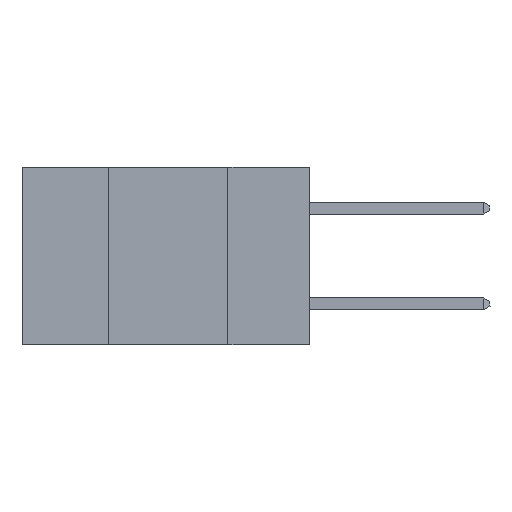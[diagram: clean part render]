
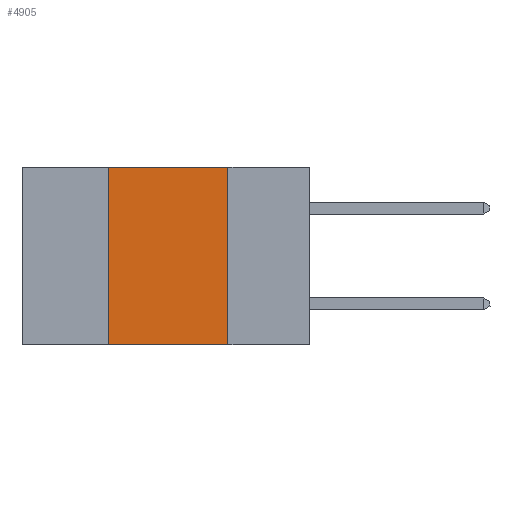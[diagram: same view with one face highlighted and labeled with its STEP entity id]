
A CAD part, left-side view. The second image highlights one B-rep face of the part: STEP entity #4905.
In plain terms, the highlighted planar face has unit normal (-1, 0, 0).
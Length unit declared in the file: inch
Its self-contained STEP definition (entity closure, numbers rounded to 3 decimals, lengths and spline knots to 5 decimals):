
#242 = FACE_OUTER_BOUND ( 'NONE', #3229, .T. ) ;
#1095 = CARTESIAN_POINT ( 'NONE',  ( 0., 0.42, 0. ) ) ;
#1418 = VERTEX_POINT ( 'NONE', #6916 ) ;
#1451 = CARTESIAN_POINT ( 'NONE',  ( 0., 0.42, 0. ) ) ;
#1574 = DIRECTION ( 'NONE',  ( 1., 0., 0. ) ) ;
#1758 = DIRECTION ( 'NONE',  ( 0., -1., 0. ) ) ;
#2388 = VERTEX_POINT ( 'NONE', #1095 ) ;
#2653 = DIRECTION ( 'NONE',  ( 0., -1., 0. ) ) ;
#3075 = LINE ( 'NONE', #4954, #3851 ) ;
#3144 = DIRECTION ( 'NONE',  ( 0., 0., -1. ) ) ;
#3229 = EDGE_LOOP ( 'NONE', ( #6020, #6443, #9209, #9977 ) ) ;
#3851 = VECTOR ( 'NONE', #2653, 39.37008 ) ;
#4242 = VERTEX_POINT ( 'NONE', #8302 ) ;
#4789 = EDGE_CURVE ( 'NONE', #5990, #1418, #3075, .T. ) ;
#4842 = EDGE_CURVE ( 'NONE', #4242, #1418, #7508, .T. ) ;
#4905 = ADVANCED_FACE ( 'NONE', ( #242 ), #10369, .F. ) ;
#4954 = CARTESIAN_POINT ( 'NONE',  ( 0., 0.6, -0.37 ) ) ;
#5072 = VECTOR ( 'NONE', #1758, 39.37008 ) ;
#5334 = DIRECTION ( 'NONE',  ( 0., 0., 1. ) ) ;
#5521 = CARTESIAN_POINT ( 'NONE',  ( 0., 0.6, 0. ) ) ;
#5676 = EDGE_CURVE ( 'NONE', #5990, #2388, #7867, .T. ) ;
#5990 = VERTEX_POINT ( 'NONE', #9290 ) ;
#6020 = ORIENTED_EDGE ( 'NONE', *, *, #4842, .F. ) ;
#6051 = CARTESIAN_POINT ( 'NONE',  ( 0., 0.17, 0. ) ) ;
#6443 = ORIENTED_EDGE ( 'NONE', *, *, #6660, .F. ) ;
#6660 = EDGE_CURVE ( 'NONE', #2388, #4242, #9333, .T. ) ;
#6916 = CARTESIAN_POINT ( 'NONE',  ( 0., 0.17, -0.37 ) ) ;
#7105 = VECTOR ( 'NONE', #5334, 39.37008 ) ;
#7508 = LINE ( 'NONE', #6051, #7756 ) ;
#7756 = VECTOR ( 'NONE', #8416, 39.37008 ) ;
#7867 = LINE ( 'NONE', #1451, #7105 ) ;
#8302 = CARTESIAN_POINT ( 'NONE',  ( 0., 0.17, 0. ) ) ;
#8416 = DIRECTION ( 'NONE',  ( 0., 0., -1. ) ) ;
#9209 = ORIENTED_EDGE ( 'NONE', *, *, #5676, .F. ) ;
#9261 = AXIS2_PLACEMENT_3D ( 'NONE', #5521, #1574, #3144 ) ;
#9290 = CARTESIAN_POINT ( 'NONE',  ( 0., 0.42, -0.37 ) ) ;
#9333 = LINE ( 'NONE', #9740, #5072 ) ;
#9740 = CARTESIAN_POINT ( 'NONE',  ( 0., 0.6, 0. ) ) ;
#9977 = ORIENTED_EDGE ( 'NONE', *, *, #4789, .T. ) ;
#10369 = PLANE ( 'NONE',  #9261 ) ;
